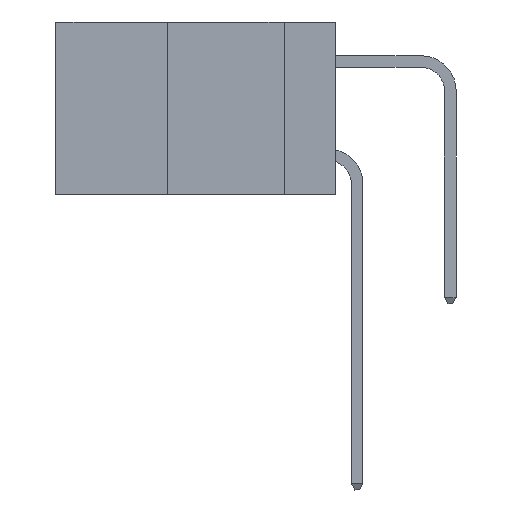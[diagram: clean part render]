
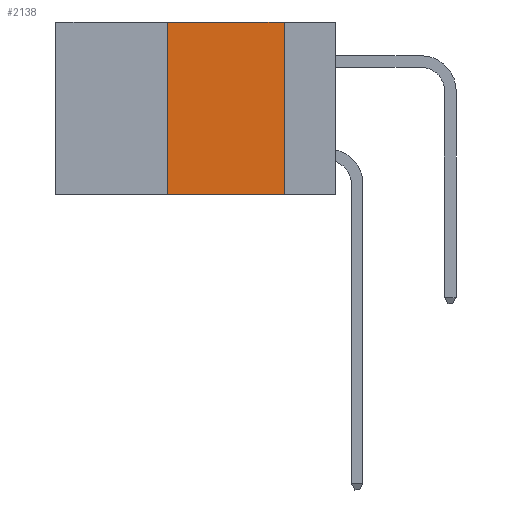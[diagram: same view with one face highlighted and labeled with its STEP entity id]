
A CAD part, left-side view. The second image highlights one B-rep face of the part: STEP entity #2138.
In plain terms, the highlighted planar face has unit normal (-1, 0, 0).
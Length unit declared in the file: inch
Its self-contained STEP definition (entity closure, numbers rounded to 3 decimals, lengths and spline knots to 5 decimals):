
#2138 = ADVANCED_FACE ( 'NONE', ( #4455 ), #9859, .F. ) ;
#2769 = CARTESIAN_POINT ( 'NONE',  ( 0., 0.36, 0. ) ) ;
#3811 = VERTEX_POINT ( 'NONE', #9874 ) ;
#3926 = DIRECTION ( 'NONE',  ( 0., 0., -1. ) ) ;
#4203 = DIRECTION ( 'NONE',  ( 0., 0., -1. ) ) ;
#4455 = FACE_OUTER_BOUND ( 'NONE', #18016, .T. ) ;
#6315 = VERTEX_POINT ( 'NONE', #17242 ) ;
#6521 = VECTOR ( 'NONE', #4203, 39.37008 ) ;
#6936 = CARTESIAN_POINT ( 'NONE',  ( 0., 0.6, 0. ) ) ;
#7179 = DIRECTION ( 'NONE',  ( 0., -1., 0. ) ) ;
#7225 = CARTESIAN_POINT ( 'NONE',  ( 0., 0.6, -0.37 ) ) ;
#7400 = LINE ( 'NONE', #7225, #14042 ) ;
#7905 = CARTESIAN_POINT ( 'NONE',  ( 0., 0.36, 0. ) ) ;
#8716 = DIRECTION ( 'NONE',  ( 0., -1., 0. ) ) ;
#9093 = LINE ( 'NONE', #13294, #6521 ) ;
#9859 = PLANE ( 'NONE',  #18291 ) ;
#9874 = CARTESIAN_POINT ( 'NONE',  ( 0., 0.36, -0.37 ) ) ;
#10106 = CARTESIAN_POINT ( 'NONE',  ( 0., 0.6, 0. ) ) ;
#11241 = ORIENTED_EDGE ( 'NONE', *, *, #17817, .T. ) ;
#11591 = VERTEX_POINT ( 'NONE', #17314 ) ;
#11722 = EDGE_CURVE ( 'NONE', #11591, #6315, #9093, .T. ) ;
#12403 = DIRECTION ( 'NONE',  ( 0., 0., 1. ) ) ;
#12510 = LINE ( 'NONE', #10106, #14193 ) ;
#13294 = CARTESIAN_POINT ( 'NONE',  ( 0., 0.11, 0. ) ) ;
#13588 = ORIENTED_EDGE ( 'NONE', *, *, #11722, .F. ) ;
#14042 = VECTOR ( 'NONE', #8716, 39.37008 ) ;
#14193 = VECTOR ( 'NONE', #7179, 39.37008 ) ;
#14411 = VERTEX_POINT ( 'NONE', #2769 ) ;
#14656 = ORIENTED_EDGE ( 'NONE', *, *, #15668, .F. ) ;
#15668 = EDGE_CURVE ( 'NONE', #14411, #11591, #12510, .T. ) ;
#15891 = ORIENTED_EDGE ( 'NONE', *, *, #19266, .F. ) ;
#17242 = CARTESIAN_POINT ( 'NONE',  ( 0., 0.11, -0.37 ) ) ;
#17314 = CARTESIAN_POINT ( 'NONE',  ( 0., 0.11, 0. ) ) ;
#17404 = LINE ( 'NONE', #7905, #18336 ) ;
#17500 = DIRECTION ( 'NONE',  ( 1., 0., 0. ) ) ;
#17817 = EDGE_CURVE ( 'NONE', #3811, #6315, #7400, .T. ) ;
#18016 = EDGE_LOOP ( 'NONE', ( #13588, #14656, #15891, #11241 ) ) ;
#18291 = AXIS2_PLACEMENT_3D ( 'NONE', #6936, #17500, #3926 ) ;
#18336 = VECTOR ( 'NONE', #12403, 39.37008 ) ;
#19266 = EDGE_CURVE ( 'NONE', #3811, #14411, #17404, .T. ) ;
